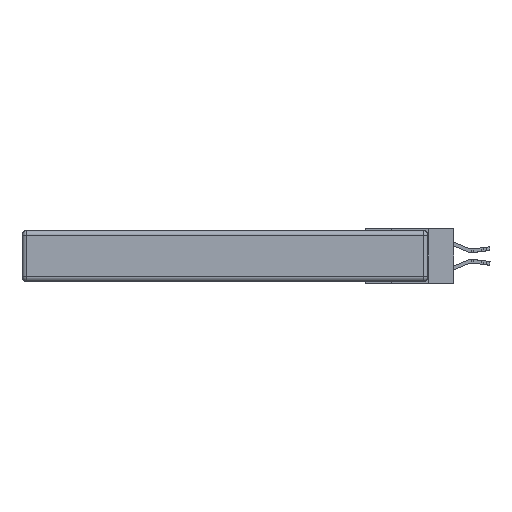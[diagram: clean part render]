
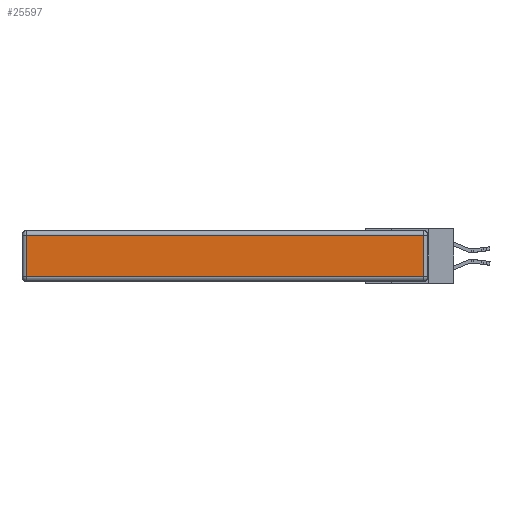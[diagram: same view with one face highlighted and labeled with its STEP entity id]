
A CAD part, left-side view. The second image highlights one B-rep face of the part: STEP entity #25597.
In plain terms, the highlighted planar face has unit normal (-1, 0, 0).
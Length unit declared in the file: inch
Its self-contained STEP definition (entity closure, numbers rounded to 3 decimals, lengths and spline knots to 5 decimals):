
#634 = CARTESIAN_POINT ( 'NONE',  ( 0., 0., -0.313 ) ) ;
#1348 = VERTEX_POINT ( 'NONE', #16326 ) ;
#1509 = ORIENTED_EDGE ( 'NONE', *, *, #1977, .T. ) ;
#1551 = LINE ( 'NONE', #634, #29730 ) ;
#1977 = EDGE_CURVE ( 'NONE', #3719, #9247, #1551, .T. ) ;
#2996 = PLANE ( 'NONE',  #10024 ) ;
#3719 = VERTEX_POINT ( 'NONE', #11866 ) ;
#7164 = VECTOR ( 'NONE', #30977, 39.37008 ) ;
#8455 = DIRECTION ( 'NONE',  ( 0., 1., 0. ) ) ;
#9247 = VERTEX_POINT ( 'NONE', #17613 ) ;
#10024 = AXIS2_PLACEMENT_3D ( 'NONE', #12622, #20237, #15015 ) ;
#10662 = CARTESIAN_POINT ( 'NONE',  ( 0., 2.72, -0.03 ) ) ;
#11110 = CARTESIAN_POINT ( 'NONE',  ( 0., 0.03, -0.343 ) ) ;
#11444 = DIRECTION ( 'NONE',  ( 0., 0., 1. ) ) ;
#11588 = EDGE_CURVE ( 'NONE', #9247, #1348, #21213, .T. ) ;
#11866 = CARTESIAN_POINT ( 'NONE',  ( 0., 2.72, -0.313 ) ) ;
#12479 = EDGE_CURVE ( 'NONE', #16823, #3719, #17595, .T. ) ;
#12622 = CARTESIAN_POINT ( 'NONE',  ( 0., 0., -0.343 ) ) ;
#12778 = ORIENTED_EDGE ( 'NONE', *, *, #11588, .T. ) ;
#13473 = FACE_OUTER_BOUND ( 'NONE', #26765, .T. ) ;
#15015 = DIRECTION ( 'NONE',  ( 0., 0., 1. ) ) ;
#15395 = DIRECTION ( 'NONE',  ( 0., -1., 0. ) ) ;
#16254 = VECTOR ( 'NONE', #11444, 39.37008 ) ;
#16283 = LINE ( 'NONE', #23501, #29761 ) ;
#16326 = CARTESIAN_POINT ( 'NONE',  ( 0., 0.03, -0.03 ) ) ;
#16529 = EDGE_CURVE ( 'NONE', #1348, #16823, #16283, .T. ) ;
#16823 = VERTEX_POINT ( 'NONE', #10662 ) ;
#17595 = LINE ( 'NONE', #28864, #7164 ) ;
#17613 = CARTESIAN_POINT ( 'NONE',  ( 0., 0.03, -0.313 ) ) ;
#20237 = DIRECTION ( 'NONE',  ( -1., 0., 0. ) ) ;
#20485 = ORIENTED_EDGE ( 'NONE', *, *, #12479, .T. ) ;
#21213 = LINE ( 'NONE', #11110, #16254 ) ;
#23501 = CARTESIAN_POINT ( 'NONE',  ( 0., 2.75, -0.03 ) ) ;
#25323 = ORIENTED_EDGE ( 'NONE', *, *, #16529, .T. ) ;
#25597 = ADVANCED_FACE ( 'NONE', ( #13473 ), #2996, .T. ) ;
#26765 = EDGE_LOOP ( 'NONE', ( #1509, #12778, #25323, #20485 ) ) ;
#28864 = CARTESIAN_POINT ( 'NONE',  ( 0., 2.72, -0.343 ) ) ;
#29730 = VECTOR ( 'NONE', #15395, 39.37008 ) ;
#29761 = VECTOR ( 'NONE', #8455, 39.37008 ) ;
#30977 = DIRECTION ( 'NONE',  ( 0., 0., -1. ) ) ;
